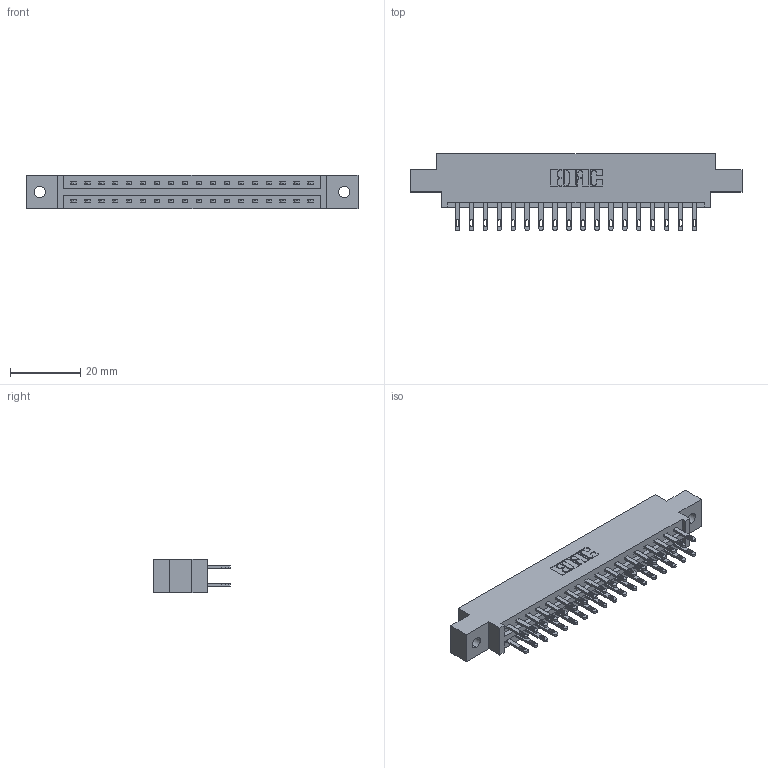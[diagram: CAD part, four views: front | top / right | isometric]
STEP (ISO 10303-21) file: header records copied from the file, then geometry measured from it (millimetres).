
FILE_DESCRIPTION (( 'STEP AP203' ), '1' );
FILE_NAME ('887-036-500-802.STEP', '2020-09-20T22:22:30', ( '' ), ( '' ), 'SwSTEP 2.0', 'SolidWorks 2020', '' );
FILE_SCHEMA (( 'CONFIG_CONTROL_DESIGN' ));
Length unit declared in the file: inch
Products named in the file (3): 345-292-001_345-293-100; 837 Part_0.170 Offset - 0.128 Dia; 887-036-500-802
Assembly tree (37 placements, depth 2):
  887-036-500-802
    837 Part_0.170 Offset - 0.128 Dia
    345-292-001_345-293-100  x36
Bounding box: 94.34 x 21.85 x 9.4 mm (x, y, z)
Volume: 9578.2 mm3; surface area: 10829.6 mm2
Topology: 37 solids, 37 shells, 1918 faces, 5831 edges, 3886 vertices
Faces by surface type: plane 1226, cylinder 692
Entity records: 17125 total; most frequent: CARTESIAN_POINT 2906, ORIENTED_EDGE 2842, DIRECTION 2517, EDGE_CURVE 1421, LINE 1289, VECTOR 1289, VERTEX_POINT 946, AXIS2_PLACEMENT_3D 614
